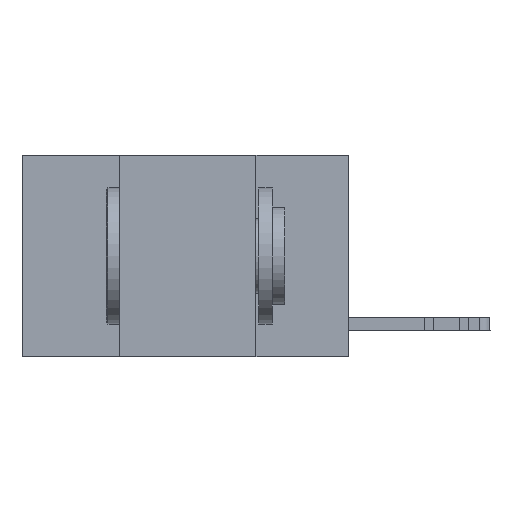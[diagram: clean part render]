
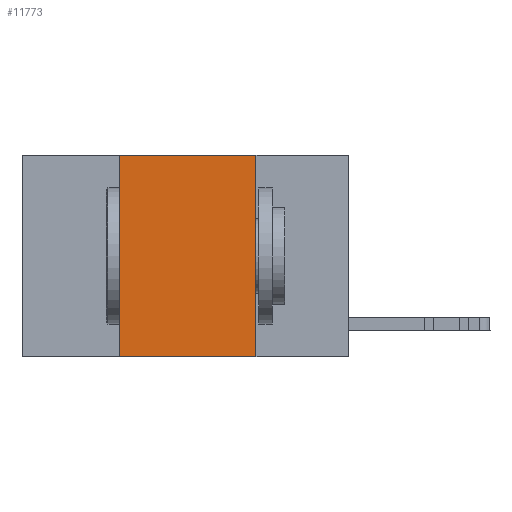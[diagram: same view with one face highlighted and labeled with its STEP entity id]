
A CAD part, left-side view. The second image highlights one B-rep face of the part: STEP entity #11773.
In plain terms, the highlighted planar face has unit normal (-1, 0, 0).
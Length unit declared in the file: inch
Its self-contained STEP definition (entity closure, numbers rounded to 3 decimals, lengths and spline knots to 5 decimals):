
#260 = DIRECTION ( 'NONE',  ( 0., -1., 0. ) ) ;
#958 = ORIENTED_EDGE ( 'NONE', *, *, #2218, .T. ) ;
#1233 = VECTOR ( 'NONE', #17114, 39.37008 ) ;
#1911 = CARTESIAN_POINT ( 'NONE',  ( 0., 0.42, -0.37 ) ) ;
#2016 = ORIENTED_EDGE ( 'NONE', *, *, #12794, .F. ) ;
#2218 = EDGE_CURVE ( 'NONE', #16741, #4543, #4869, .T. ) ;
#2414 = CARTESIAN_POINT ( 'NONE',  ( 0., 0.6, 0. ) ) ;
#2507 = VECTOR ( 'NONE', #20104, 39.37008 ) ;
#2750 = LINE ( 'NONE', #22130, #2507 ) ;
#2759 = DIRECTION ( 'NONE',  ( 0., -1., 0. ) ) ;
#3390 = CARTESIAN_POINT ( 'NONE',  ( 0., 0.17, -0.37 ) ) ;
#3906 = CARTESIAN_POINT ( 'NONE',  ( 0., 0.17, 0. ) ) ;
#4543 = VERTEX_POINT ( 'NONE', #3390 ) ;
#4825 = EDGE_LOOP ( 'NONE', ( #2016, #26309, #21541, #958 ) ) ;
#4869 = LINE ( 'NONE', #13525, #13746 ) ;
#5001 = CARTESIAN_POINT ( 'NONE',  ( 0., 0.6, 0. ) ) ;
#5869 = CARTESIAN_POINT ( 'NONE',  ( 0., 0.17, 0. ) ) ;
#6223 = CARTESIAN_POINT ( 'NONE',  ( 0., 0.42, 0. ) ) ;
#9492 = EDGE_CURVE ( 'NONE', #16741, #22960, #2750, .T. ) ;
#11667 = DIRECTION ( 'NONE',  ( 0., 0., -1. ) ) ;
#11773 = ADVANCED_FACE ( 'NONE', ( #17951 ), #24545, .F. ) ;
#12794 = EDGE_CURVE ( 'NONE', #14074, #4543, #23553, .T. ) ;
#13525 = CARTESIAN_POINT ( 'NONE',  ( 0., 0.6, -0.37 ) ) ;
#13746 = VECTOR ( 'NONE', #2759, 39.37008 ) ;
#14074 = VERTEX_POINT ( 'NONE', #3906 ) ;
#16741 = VERTEX_POINT ( 'NONE', #1911 ) ;
#17114 = DIRECTION ( 'NONE',  ( 0., 0., -1. ) ) ;
#17951 = FACE_OUTER_BOUND ( 'NONE', #4825, .T. ) ;
#18834 = EDGE_CURVE ( 'NONE', #22960, #14074, #24341, .T. ) ;
#20104 = DIRECTION ( 'NONE',  ( 0., 0., 1. ) ) ;
#21541 = ORIENTED_EDGE ( 'NONE', *, *, #9492, .F. ) ;
#22130 = CARTESIAN_POINT ( 'NONE',  ( 0., 0.42, 0. ) ) ;
#22548 = DIRECTION ( 'NONE',  ( 1., 0., 0. ) ) ;
#22960 = VERTEX_POINT ( 'NONE', #6223 ) ;
#23553 = LINE ( 'NONE', #5869, #1233 ) ;
#24341 = LINE ( 'NONE', #2414, #25065 ) ;
#24545 = PLANE ( 'NONE',  #26677 ) ;
#25065 = VECTOR ( 'NONE', #260, 39.37008 ) ;
#26309 = ORIENTED_EDGE ( 'NONE', *, *, #18834, .F. ) ;
#26677 = AXIS2_PLACEMENT_3D ( 'NONE', #5001, #22548, #11667 ) ;
